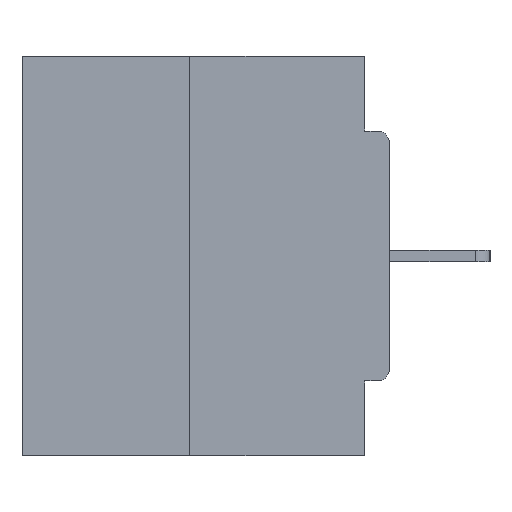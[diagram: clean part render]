
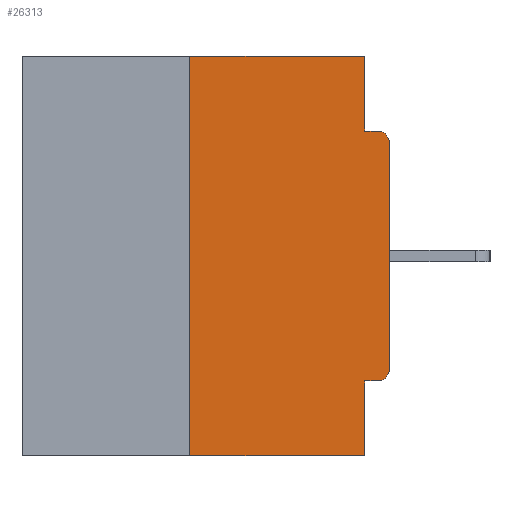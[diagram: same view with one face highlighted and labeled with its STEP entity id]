
A CAD part, left-side view. The second image highlights one B-rep face of the part: STEP entity #26313.
In plain terms, the highlighted planar face has unit normal (-1, 0, 0).
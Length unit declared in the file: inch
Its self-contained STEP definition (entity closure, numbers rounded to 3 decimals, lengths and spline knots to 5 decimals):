
#20 = DIRECTION ( 'NONE',  ( 0., -1., 0. ) ) ;
#1139 = EDGE_CURVE ( 'NONE', #2429, #27556, #20626, .T. ) ;
#2133 = CARTESIAN_POINT ( 'NONE',  ( 0., 0.031, -0.4065 ) ) ;
#2429 = VERTEX_POINT ( 'NONE', #2133 ) ;
#2431 = EDGE_CURVE ( 'NONE', #5404, #20081, #7357, .T. ) ;
#2630 = LINE ( 'NONE', #17018, #31146 ) ;
#2853 = LINE ( 'NONE', #3010, #3720 ) ;
#3003 = EDGE_CURVE ( 'NONE', #29129, #11252, #2853, .T. ) ;
#3010 = CARTESIAN_POINT ( 'NONE',  ( 0., 0., -0.0935 ) ) ;
#3079 = AXIS2_PLACEMENT_3D ( 'NONE', #22538, #3360, #13088 ) ;
#3360 = DIRECTION ( 'NONE',  ( -1., 0., 0. ) ) ;
#3658 = DIRECTION ( 'NONE',  ( 0., 0., -1. ) ) ;
#3670 = DIRECTION ( 'NONE',  ( 0., 0., -1. ) ) ;
#3720 = VECTOR ( 'NONE', #20, 39.37008 ) ;
#3955 = ORIENTED_EDGE ( 'NONE', *, *, #10055, .T. ) ;
#4196 = ORIENTED_EDGE ( 'NONE', *, *, #26838, .F. ) ;
#4528 = CARTESIAN_POINT ( 'NONE',  ( 0., 0.015, -0.1085 ) ) ;
#5194 = CARTESIAN_POINT ( 'NONE',  ( 0., 0.031, 0. ) ) ;
#5404 = VERTEX_POINT ( 'NONE', #14067 ) ;
#6451 = CARTESIAN_POINT ( 'NONE',  ( 0., 0.015, -0.0935 ) ) ;
#6711 = VERTEX_POINT ( 'NONE', #15226 ) ;
#6758 = DIRECTION ( 'NONE',  ( 0., 0., -1. ) ) ;
#6970 = CARTESIAN_POINT ( 'NONE',  ( 0., 0.46, 0. ) ) ;
#6990 = CARTESIAN_POINT ( 'NONE',  ( 0., 0.25, -0.5 ) ) ;
#7044 = CARTESIAN_POINT ( 'NONE',  ( 0., 0., 0. ) ) ;
#7061 = VECTOR ( 'NONE', #12913, 39.37008 ) ;
#7357 = LINE ( 'NONE', #7044, #22085 ) ;
#7885 = CIRCLE ( 'NONE', #25755, 0.015 ) ;
#8041 = CARTESIAN_POINT ( 'NONE',  ( 0., 0.25, 0. ) ) ;
#8600 = ORIENTED_EDGE ( 'NONE', *, *, #27886, .T. ) ;
#9348 = DIRECTION ( 'NONE',  ( 0., -1., 0. ) ) ;
#10055 = EDGE_CURVE ( 'NONE', #6711, #5404, #28047, .T. ) ;
#11069 = VECTOR ( 'NONE', #9348, 39.37008 ) ;
#11252 = VERTEX_POINT ( 'NONE', #6451 ) ;
#11471 = DIRECTION ( 'NONE',  ( 1., 0., 0. ) ) ;
#12913 = DIRECTION ( 'NONE',  ( 0., -1., 0. ) ) ;
#13088 = DIRECTION ( 'NONE',  ( 0., 0., -1. ) ) ;
#13729 = ORIENTED_EDGE ( 'NONE', *, *, #1139, .F. ) ;
#13790 = CARTESIAN_POINT ( 'NONE',  ( 0., 0., -0.1085 ) ) ;
#13822 = ORIENTED_EDGE ( 'NONE', *, *, #22682, .T. ) ;
#13892 = FACE_OUTER_BOUND ( 'NONE', #15452, .T. ) ;
#14067 = CARTESIAN_POINT ( 'NONE',  ( 0., 0., -0.3915 ) ) ;
#14795 = DIRECTION ( 'NONE',  ( 0., 0., -1. ) ) ;
#15083 = LINE ( 'NONE', #15714, #27085 ) ;
#15226 = CARTESIAN_POINT ( 'NONE',  ( 0., 0.015, -0.4065 ) ) ;
#15416 = EDGE_CURVE ( 'NONE', #6711, #2429, #2630, .T. ) ;
#15452 = EDGE_LOOP ( 'NONE', ( #4196, #27238, #8600, #13729, #21874, #3955, #18135, #13822, #24704, #18535 ) ) ;
#15714 = CARTESIAN_POINT ( 'NONE',  ( 0., 0.25, 0. ) ) ;
#15817 = PLANE ( 'NONE',  #25359 ) ;
#16267 = EDGE_CURVE ( 'NONE', #30970, #29129, #17526, .T. ) ;
#17018 = CARTESIAN_POINT ( 'NONE',  ( 0., 0., -0.4065 ) ) ;
#17526 = LINE ( 'NONE', #5194, #24565 ) ;
#18135 = ORIENTED_EDGE ( 'NONE', *, *, #2431, .T. ) ;
#18535 = ORIENTED_EDGE ( 'NONE', *, *, #16267, .F. ) ;
#18694 = EDGE_CURVE ( 'NONE', #19259, #26930, #15083, .T. ) ;
#18728 = CARTESIAN_POINT ( 'NONE',  ( 0., 0.031, -0.5 ) ) ;
#19259 = VERTEX_POINT ( 'NONE', #6990 ) ;
#20081 = VERTEX_POINT ( 'NONE', #13790 ) ;
#20626 = LINE ( 'NONE', #27463, #23502 ) ;
#21874 = ORIENTED_EDGE ( 'NONE', *, *, #15416, .F. ) ;
#22085 = VECTOR ( 'NONE', #28918, 39.37008 ) ;
#22538 = CARTESIAN_POINT ( 'NONE',  ( 0., 0.015, -0.3915 ) ) ;
#22682 = EDGE_CURVE ( 'NONE', #20081, #11252, #7885, .T. ) ;
#23302 = CARTESIAN_POINT ( 'NONE',  ( 0., 0.46, 0. ) ) ;
#23502 = VECTOR ( 'NONE', #3658, 39.37008 ) ;
#23605 = CARTESIAN_POINT ( 'NONE',  ( 0., 0.031, 0. ) ) ;
#24565 = VECTOR ( 'NONE', #14795, 39.37008 ) ;
#24704 = ORIENTED_EDGE ( 'NONE', *, *, #3003, .F. ) ;
#25040 = CARTESIAN_POINT ( 'NONE',  ( 0., 0.46, -0.5 ) ) ;
#25353 = LINE ( 'NONE', #25040, #7061 ) ;
#25359 = AXIS2_PLACEMENT_3D ( 'NONE', #23302, #11471, #3670 ) ;
#25440 = DIRECTION ( 'NONE',  ( 0., 0., 1. ) ) ;
#25755 = AXIS2_PLACEMENT_3D ( 'NONE', #4528, #28640, #6758 ) ;
#26313 = ADVANCED_FACE ( 'NONE', ( #13892 ), #15817, .F. ) ;
#26838 = EDGE_CURVE ( 'NONE', #26930, #30970, #28705, .T. ) ;
#26930 = VERTEX_POINT ( 'NONE', #8041 ) ;
#27030 = DIRECTION ( 'NONE',  ( 0., 1., 0. ) ) ;
#27085 = VECTOR ( 'NONE', #25440, 39.37008 ) ;
#27238 = ORIENTED_EDGE ( 'NONE', *, *, #18694, .F. ) ;
#27463 = CARTESIAN_POINT ( 'NONE',  ( 0., 0.031, -0.5 ) ) ;
#27556 = VERTEX_POINT ( 'NONE', #18728 ) ;
#27886 = EDGE_CURVE ( 'NONE', #19259, #27556, #25353, .T. ) ;
#28047 = CIRCLE ( 'NONE', #3079, 0.015 ) ;
#28640 = DIRECTION ( 'NONE',  ( -1., 0., 0. ) ) ;
#28705 = LINE ( 'NONE', #6970, #11069 ) ;
#28918 = DIRECTION ( 'NONE',  ( 0., 0., 1. ) ) ;
#29129 = VERTEX_POINT ( 'NONE', #30468 ) ;
#30468 = CARTESIAN_POINT ( 'NONE',  ( 0., 0.031, -0.0935 ) ) ;
#30970 = VERTEX_POINT ( 'NONE', #23605 ) ;
#31146 = VECTOR ( 'NONE', #27030, 39.37008 ) ;
